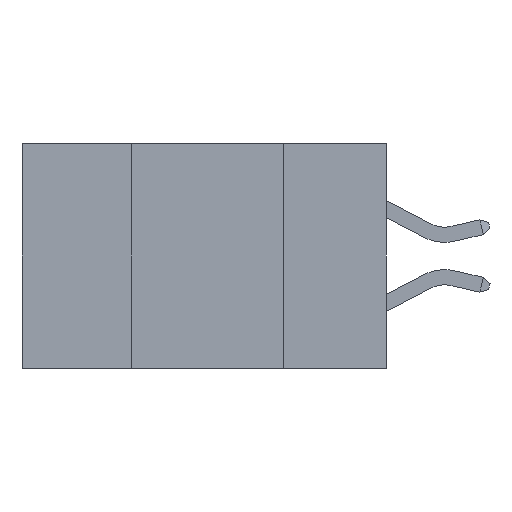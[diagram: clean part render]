
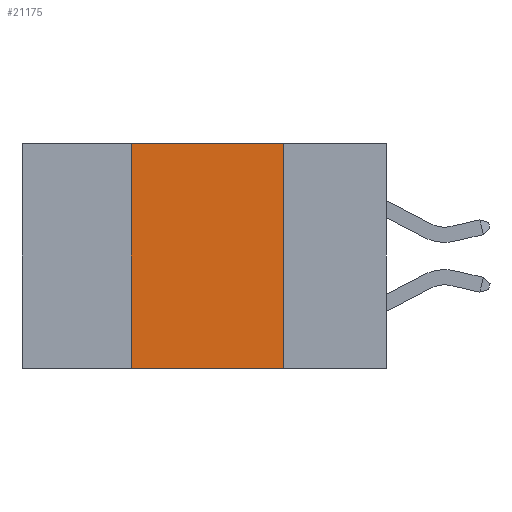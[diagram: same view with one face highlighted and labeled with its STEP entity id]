
A CAD part, left-side view. The second image highlights one B-rep face of the part: STEP entity #21175.
In plain terms, the highlighted planar face has unit normal (-1, 0, 0).
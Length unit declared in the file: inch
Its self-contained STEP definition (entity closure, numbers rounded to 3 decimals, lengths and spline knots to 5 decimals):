
#552 = CARTESIAN_POINT ( 'NONE',  ( 0., 0.6, 0. ) ) ;
#1191 = DIRECTION ( 'NONE',  ( 1., 0., 0. ) ) ;
#1618 = EDGE_CURVE ( 'NONE', #10075, #1935, #6770, .T. ) ;
#1935 = VERTEX_POINT ( 'NONE', #19331 ) ;
#2263 = DIRECTION ( 'NONE',  ( 0., -1., 0. ) ) ;
#3040 = FACE_OUTER_BOUND ( 'NONE', #19439, .T. ) ;
#3275 = EDGE_CURVE ( 'NONE', #9988, #16720, #10457, .T. ) ;
#3652 = CARTESIAN_POINT ( 'NONE',  ( 0., 0.42, -0.37 ) ) ;
#5445 = CARTESIAN_POINT ( 'NONE',  ( 0., 0.6, -0.37 ) ) ;
#6107 = EDGE_CURVE ( 'NONE', #16720, #10075, #17572, .T. ) ;
#6770 = LINE ( 'NONE', #18834, #19903 ) ;
#8125 = CARTESIAN_POINT ( 'NONE',  ( 0., 0.42, -0.37 ) ) ;
#8635 = ORIENTED_EDGE ( 'NONE', *, *, #1618, .F. ) ;
#9534 = EDGE_CURVE ( 'NONE', #9988, #1935, #14674, .T. ) ;
#9724 = VECTOR ( 'NONE', #15394, 39.37008 ) ;
#9988 = VERTEX_POINT ( 'NONE', #8125 ) ;
#10075 = VERTEX_POINT ( 'NONE', #18253 ) ;
#10457 = LINE ( 'NONE', #3652, #14877 ) ;
#12015 = ORIENTED_EDGE ( 'NONE', *, *, #6107, .F. ) ;
#12840 = DIRECTION ( 'NONE',  ( 0., 0., -1. ) ) ;
#13463 = ORIENTED_EDGE ( 'NONE', *, *, #3275, .F. ) ;
#14674 = LINE ( 'NONE', #5445, #9724 ) ;
#14877 = VECTOR ( 'NONE', #15284, 39.37008 ) ;
#15284 = DIRECTION ( 'NONE',  ( 0., 0., 1. ) ) ;
#15394 = DIRECTION ( 'NONE',  ( 0., -1., 0. ) ) ;
#16720 = VERTEX_POINT ( 'NONE', #19189 ) ;
#16949 = ORIENTED_EDGE ( 'NONE', *, *, #9534, .T. ) ;
#17063 = VECTOR ( 'NONE', #2263, 39.37008 ) ;
#17572 = LINE ( 'NONE', #552, #17063 ) ;
#18253 = CARTESIAN_POINT ( 'NONE',  ( 0., 0.17, 0. ) ) ;
#18707 = AXIS2_PLACEMENT_3D ( 'NONE', #19360, #1191, #12840 ) ;
#18834 = CARTESIAN_POINT ( 'NONE',  ( 0., 0.17, -0.37 ) ) ;
#19098 = DIRECTION ( 'NONE',  ( 0., 0., -1. ) ) ;
#19189 = CARTESIAN_POINT ( 'NONE',  ( 0., 0.42, 0. ) ) ;
#19331 = CARTESIAN_POINT ( 'NONE',  ( 0., 0.17, -0.37 ) ) ;
#19360 = CARTESIAN_POINT ( 'NONE',  ( 0., 0.6, 0. ) ) ;
#19439 = EDGE_LOOP ( 'NONE', ( #8635, #12015, #13463, #16949 ) ) ;
#19903 = VECTOR ( 'NONE', #19098, 39.37008 ) ;
#20883 = PLANE ( 'NONE',  #18707 ) ;
#21175 = ADVANCED_FACE ( 'NONE', ( #3040 ), #20883, .F. ) ;
